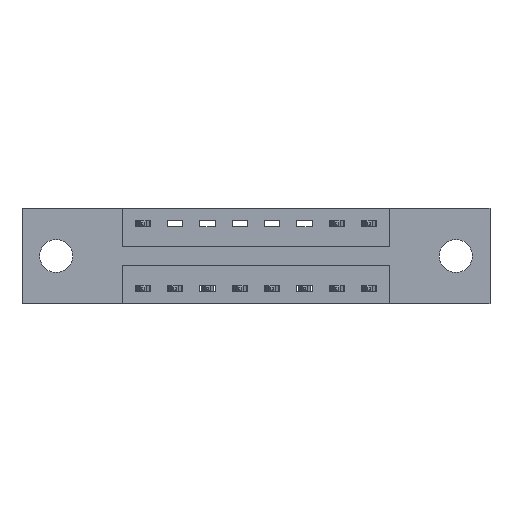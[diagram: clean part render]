
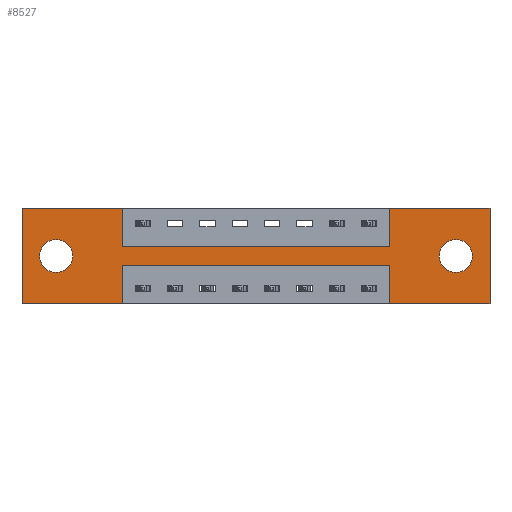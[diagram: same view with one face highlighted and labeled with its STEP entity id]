
A CAD part, front view. The second image highlights one B-rep face of the part: STEP entity #8527.
In plain terms, the highlighted planar face has unit normal (0, -1, 0).
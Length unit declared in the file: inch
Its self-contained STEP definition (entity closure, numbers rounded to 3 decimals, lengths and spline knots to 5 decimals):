
#28 = CARTESIAN_POINT ( 'NONE',  ( 0.3875, 0., 0. ) ) ;
#63 = EDGE_CURVE ( 'NONE', #8870, #3120, #2423, .T. ) ;
#86 = EDGE_CURVE ( 'NONE', #7169, #5451, #9553, .T. ) ;
#240 = DIRECTION ( 'NONE',  ( 0., 0., 1. ) ) ;
#387 = EDGE_CURVE ( 'NONE', #928, #7169, #3322, .T. ) ;
#450 = DIRECTION ( 'NONE',  ( 0., 1., 0. ) ) ;
#473 = DIRECTION ( 'NONE',  ( 0., 0., -1. ) ) ;
#522 = EDGE_CURVE ( 'NONE', #7875, #928, #5363, .T. ) ;
#853 = ORIENTED_EDGE ( 'NONE', *, *, #6447, .T. ) ;
#854 = DIRECTION ( 'NONE',  ( 0., 0., 1. ) ) ;
#928 = VERTEX_POINT ( 'NONE', #8652 ) ;
#973 = CARTESIAN_POINT ( 'NONE',  ( 0.3875, 0., -0.22 ) ) ;
#1102 = VECTOR ( 'NONE', #8435, 39.37008 ) ;
#1109 = ORIENTED_EDGE ( 'NONE', *, *, #7412, .F. ) ;
#1155 = VECTOR ( 'NONE', #4522, 39.37008 ) ;
#1450 = VERTEX_POINT ( 'NONE', #9595 ) ;
#1471 = LINE ( 'NONE', #9046, #9114 ) ;
#1610 = ORIENTED_EDGE ( 'NONE', *, *, #387, .F. ) ;
#1614 = VERTEX_POINT ( 'NONE', #6851 ) ;
#1651 = CARTESIAN_POINT ( 'NONE',  ( 1.4225, 0., -0.22 ) ) ;
#1662 = VERTEX_POINT ( 'NONE', #3089 ) ;
#1716 = EDGE_CURVE ( 'NONE', #5451, #2032, #3069, .T. ) ;
#1783 = CARTESIAN_POINT ( 'NONE',  ( 0.3875, 0., -0.37 ) ) ;
#1859 = ORIENTED_EDGE ( 'NONE', *, *, #63, .F. ) ;
#1995 = AXIS2_PLACEMENT_3D ( 'NONE', #7890, #3398, #8624 ) ;
#2032 = VERTEX_POINT ( 'NONE', #4253 ) ;
#2047 = DIRECTION ( 'NONE',  ( 0., -1., 0. ) ) ;
#2110 = VERTEX_POINT ( 'NONE', #2164 ) ;
#2164 = CARTESIAN_POINT ( 'NONE',  ( 1.6775, 0., -0.249 ) ) ;
#2169 = VECTOR ( 'NONE', #7606, 39.37008 ) ;
#2182 = VECTOR ( 'NONE', #4032, 39.37008 ) ;
#2358 = EDGE_LOOP ( 'NONE', ( #1109, #3109, #5025, #7133, #9035, #3327, #7358, #1610, #3566, #9453, #1859, #3809 ) ) ;
#2423 = LINE ( 'NONE', #7069, #4371 ) ;
#2636 = LINE ( 'NONE', #973, #2182 ) ;
#2741 = CIRCLE ( 'NONE', #1995, 0.064 ) ;
#2806 = EDGE_LOOP ( 'NONE', ( #4789, #6915 ) ) ;
#2896 = VERTEX_POINT ( 'NONE', #4835 ) ;
#3069 = LINE ( 'NONE', #3872, #6884 ) ;
#3089 = CARTESIAN_POINT ( 'NONE',  ( 0.1325, 0., -0.121 ) ) ;
#3109 = ORIENTED_EDGE ( 'NONE', *, *, #7084, .F. ) ;
#3120 = VERTEX_POINT ( 'NONE', #7361 ) ;
#3159 = LINE ( 'NONE', #5178, #1155 ) ;
#3165 = VERTEX_POINT ( 'NONE', #8846 ) ;
#3167 = CARTESIAN_POINT ( 'NONE',  ( 0.1325, 0., -0.185 ) ) ;
#3322 = LINE ( 'NONE', #9240, #1102 ) ;
#3327 = ORIENTED_EDGE ( 'NONE', *, *, #1716, .F. ) ;
#3396 = EDGE_CURVE ( 'NONE', #2032, #1614, #3159, .T. ) ;
#3398 = DIRECTION ( 'NONE',  ( 0., 1., 0. ) ) ;
#3438 = VECTOR ( 'NONE', #5985, 39.37008 ) ;
#3566 = ORIENTED_EDGE ( 'NONE', *, *, #522, .F. ) ;
#3639 = FACE_OUTER_BOUND ( 'NONE', #2358, .T. ) ;
#3809 = ORIENTED_EDGE ( 'NONE', *, *, #6432, .F. ) ;
#3872 = CARTESIAN_POINT ( 'NONE',  ( 0., 0., 0. ) ) ;
#3893 = LINE ( 'NONE', #6907, #2169 ) ;
#3927 = DIRECTION ( 'NONE',  ( 0., 0., 1. ) ) ;
#4026 = DIRECTION ( 'NONE',  ( 0., 0., -1. ) ) ;
#4032 = DIRECTION ( 'NONE',  ( -1., 0., 0. ) ) ;
#4203 = CARTESIAN_POINT ( 'NONE',  ( 0.3875, 0., 0. ) ) ;
#4253 = CARTESIAN_POINT ( 'NONE',  ( 1.81, 0., 0. ) ) ;
#4371 = VECTOR ( 'NONE', #8642, 39.37008 ) ;
#4449 = LINE ( 'NONE', #1783, #8189 ) ;
#4522 = DIRECTION ( 'NONE',  ( 0., 0., -1. ) ) ;
#4599 = AXIS2_PLACEMENT_3D ( 'NONE', #9209, #4723, #240 ) ;
#4723 = DIRECTION ( 'NONE',  ( 0., 1., 0. ) ) ;
#4789 = ORIENTED_EDGE ( 'NONE', *, *, #7238, .T. ) ;
#4835 = CARTESIAN_POINT ( 'NONE',  ( 1.6775, 0., -0.121 ) ) ;
#4928 = CARTESIAN_POINT ( 'NONE',  ( 1.6775, 0., -0.185 ) ) ;
#5025 = ORIENTED_EDGE ( 'NONE', *, *, #7209, .F. ) ;
#5036 = VERTEX_POINT ( 'NONE', #5961 ) ;
#5150 = CARTESIAN_POINT ( 'NONE',  ( 0., 0., -0.37 ) ) ;
#5178 = CARTESIAN_POINT ( 'NONE',  ( 1.81, 0., 0. ) ) ;
#5254 = CARTESIAN_POINT ( 'NONE',  ( 1.4225, 0., -0.15 ) ) ;
#5297 = DIRECTION ( 'NONE',  ( 1., 0., 0. ) ) ;
#5344 = CIRCLE ( 'NONE', #4599, 0.064 ) ;
#5363 = LINE ( 'NONE', #28, #7235 ) ;
#5451 = VERTEX_POINT ( 'NONE', #9527 ) ;
#5579 = FACE_BOUND ( 'NONE', #8946, .T. ) ;
#5611 = LINE ( 'NONE', #5628, #9336 ) ;
#5628 = CARTESIAN_POINT ( 'NONE',  ( 0., 0., -0.37 ) ) ;
#5712 = DIRECTION ( 'NONE',  ( 0., 0., -1. ) ) ;
#5961 = CARTESIAN_POINT ( 'NONE',  ( 0.3875, 0., -0.37 ) ) ;
#5985 = DIRECTION ( 'NONE',  ( -1., 0., 0. ) ) ;
#6068 = EDGE_CURVE ( 'NONE', #1614, #1450, #9549, .T. ) ;
#6256 = DIRECTION ( 'NONE',  ( 0., 0., -1. ) ) ;
#6432 = EDGE_CURVE ( 'NONE', #5036, #8870, #5611, .T. ) ;
#6447 = EDGE_CURVE ( 'NONE', #2110, #2896, #9123, .T. ) ;
#6459 = DIRECTION ( 'NONE',  ( -1., 0., 0. ) ) ;
#6617 = EDGE_CURVE ( 'NONE', #7018, #1662, #5344, .T. ) ;
#6622 = CARTESIAN_POINT ( 'NONE',  ( 1.4225, 0., 0. ) ) ;
#6636 = DIRECTION ( 'NONE',  ( 0., 0., 1. ) ) ;
#6666 = EDGE_CURVE ( 'NONE', #2896, #2110, #2741, .T. ) ;
#6851 = CARTESIAN_POINT ( 'NONE',  ( 1.81, 0., -0.37 ) ) ;
#6884 = VECTOR ( 'NONE', #5297, 39.37008 ) ;
#6905 = EDGE_CURVE ( 'NONE', #3120, #7875, #3893, .T. ) ;
#6907 = CARTESIAN_POINT ( 'NONE',  ( 0., 0., 0. ) ) ;
#6915 = ORIENTED_EDGE ( 'NONE', *, *, #6617, .T. ) ;
#7018 = VERTEX_POINT ( 'NONE', #8400 ) ;
#7069 = CARTESIAN_POINT ( 'NONE',  ( 0., 0., 0. ) ) ;
#7084 = EDGE_CURVE ( 'NONE', #7225, #3165, #2636, .T. ) ;
#7133 = ORIENTED_EDGE ( 'NONE', *, *, #6068, .F. ) ;
#7169 = VERTEX_POINT ( 'NONE', #5254 ) ;
#7209 = EDGE_CURVE ( 'NONE', #1450, #7225, #1471, .T. ) ;
#7220 = CIRCLE ( 'NONE', #9177, 0.064 ) ;
#7225 = VERTEX_POINT ( 'NONE', #1651 ) ;
#7235 = VECTOR ( 'NONE', #6256, 39.37008 ) ;
#7238 = EDGE_CURVE ( 'NONE', #1662, #7018, #7220, .T. ) ;
#7358 = ORIENTED_EDGE ( 'NONE', *, *, #86, .F. ) ;
#7361 = CARTESIAN_POINT ( 'NONE',  ( 0., 0., 0. ) ) ;
#7412 = EDGE_CURVE ( 'NONE', #3165, #5036, #4449, .T. ) ;
#7424 = FACE_BOUND ( 'NONE', #2806, .T. ) ;
#7606 = DIRECTION ( 'NONE',  ( 1., 0., 0. ) ) ;
#7673 = VECTOR ( 'NONE', #6636, 39.37008 ) ;
#7875 = VERTEX_POINT ( 'NONE', #4203 ) ;
#7890 = CARTESIAN_POINT ( 'NONE',  ( 1.6775, 0., -0.185 ) ) ;
#8189 = VECTOR ( 'NONE', #4026, 39.37008 ) ;
#8364 = DIRECTION ( 'NONE',  ( 0., 1., 0. ) ) ;
#8400 = CARTESIAN_POINT ( 'NONE',  ( 0.1325, 0., -0.249 ) ) ;
#8435 = DIRECTION ( 'NONE',  ( 1., 0., 0. ) ) ;
#8527 = ADVANCED_FACE ( 'NONE', ( #5579, #7424, #3639 ), #9407, .T. ) ;
#8581 = ORIENTED_EDGE ( 'NONE', *, *, #6666, .T. ) ;
#8624 = DIRECTION ( 'NONE',  ( 0., 0., -1. ) ) ;
#8642 = DIRECTION ( 'NONE',  ( 0., 0., 1. ) ) ;
#8652 = CARTESIAN_POINT ( 'NONE',  ( 0.3875, 0., -0.15 ) ) ;
#8730 = CARTESIAN_POINT ( 'NONE',  ( 0., 0., -0.37 ) ) ;
#8846 = CARTESIAN_POINT ( 'NONE',  ( 0.3875, 0., -0.22 ) ) ;
#8852 = CARTESIAN_POINT ( 'NONE',  ( 0., 0., -0.37 ) ) ;
#8870 = VERTEX_POINT ( 'NONE', #8852 ) ;
#8946 = EDGE_LOOP ( 'NONE', ( #8581, #853 ) ) ;
#9035 = ORIENTED_EDGE ( 'NONE', *, *, #3396, .F. ) ;
#9046 = CARTESIAN_POINT ( 'NONE',  ( 1.4225, 0., -0.37 ) ) ;
#9114 = VECTOR ( 'NONE', #854, 39.37008 ) ;
#9123 = CIRCLE ( 'NONE', #9609, 0.064 ) ;
#9177 = AXIS2_PLACEMENT_3D ( 'NONE', #3167, #8364, #3927 ) ;
#9209 = CARTESIAN_POINT ( 'NONE',  ( 0.1325, 0., -0.185 ) ) ;
#9240 = CARTESIAN_POINT ( 'NONE',  ( 0.3875, 0., -0.15 ) ) ;
#9336 = VECTOR ( 'NONE', #6459, 39.37008 ) ;
#9402 = AXIS2_PLACEMENT_3D ( 'NONE', #8730, #2047, #473 ) ;
#9407 = PLANE ( 'NONE',  #9402 ) ;
#9453 = ORIENTED_EDGE ( 'NONE', *, *, #6905, .F. ) ;
#9527 = CARTESIAN_POINT ( 'NONE',  ( 1.4225, 0., 0. ) ) ;
#9549 = LINE ( 'NONE', #5150, #3438 ) ;
#9553 = LINE ( 'NONE', #6622, #7673 ) ;
#9595 = CARTESIAN_POINT ( 'NONE',  ( 1.4225, 0., -0.37 ) ) ;
#9609 = AXIS2_PLACEMENT_3D ( 'NONE', #4928, #450, #5712 ) ;
